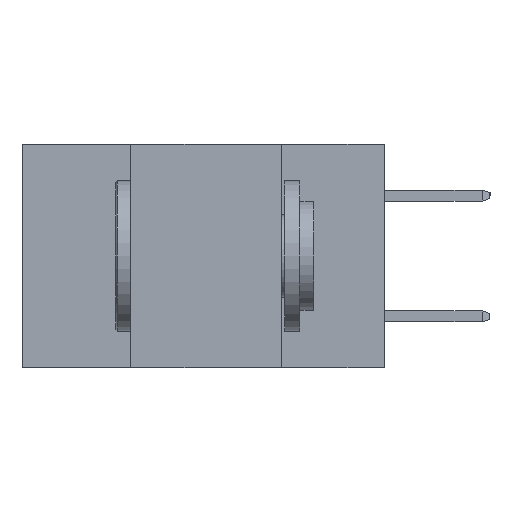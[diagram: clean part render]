
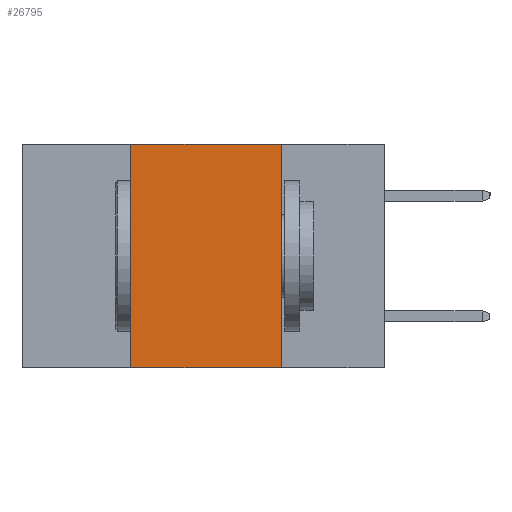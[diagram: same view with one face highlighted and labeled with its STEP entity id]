
A CAD part, left-side view. The second image highlights one B-rep face of the part: STEP entity #26795.
In plain terms, the highlighted planar face has unit normal (-1, 0, 0).
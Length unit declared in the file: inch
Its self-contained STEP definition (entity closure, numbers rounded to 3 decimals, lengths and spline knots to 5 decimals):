
#419 = CARTESIAN_POINT ( 'NONE',  ( 0., 0.17, -0.37 ) ) ;
#626 = VECTOR ( 'NONE', #10314, 39.37008 ) ;
#770 = DIRECTION ( 'NONE',  ( 0., 0., -1. ) ) ;
#1267 = EDGE_LOOP ( 'NONE', ( #12982, #4281, #22474, #10331 ) ) ;
#1413 = VECTOR ( 'NONE', #6428, 39.37008 ) ;
#2016 = VECTOR ( 'NONE', #3237, 39.37008 ) ;
#3237 = DIRECTION ( 'NONE',  ( 0., 0., -1. ) ) ;
#4281 = ORIENTED_EDGE ( 'NONE', *, *, #20757, .F. ) ;
#4662 = EDGE_CURVE ( 'NONE', #10327, #23945, #9200, .T. ) ;
#4776 = VECTOR ( 'NONE', #5690, 39.37008 ) ;
#4963 = FACE_OUTER_BOUND ( 'NONE', #1267, .T. ) ;
#5690 = DIRECTION ( 'NONE',  ( 0., 0., 1. ) ) ;
#6217 = LINE ( 'NONE', #24453, #4776 ) ;
#6428 = DIRECTION ( 'NONE',  ( 0., -1., 0. ) ) ;
#6830 = CARTESIAN_POINT ( 'NONE',  ( 0., 0.6, -0.37 ) ) ;
#9200 = LINE ( 'NONE', #15189, #2016 ) ;
#10174 = CARTESIAN_POINT ( 'NONE',  ( 0., 0.6, 0. ) ) ;
#10314 = DIRECTION ( 'NONE',  ( 0., -1., 0. ) ) ;
#10327 = VERTEX_POINT ( 'NONE', #24764 ) ;
#10331 = ORIENTED_EDGE ( 'NONE', *, *, #12918, .T. ) ;
#10918 = CARTESIAN_POINT ( 'NONE',  ( 0., 0.42, -0.37 ) ) ;
#12217 = CARTESIAN_POINT ( 'NONE',  ( 0., 0.42, 0. ) ) ;
#12918 = EDGE_CURVE ( 'NONE', #22150, #23945, #21374, .T. ) ;
#12982 = ORIENTED_EDGE ( 'NONE', *, *, #4662, .F. ) ;
#15034 = DIRECTION ( 'NONE',  ( 1., 0., 0. ) ) ;
#15127 = VERTEX_POINT ( 'NONE', #12217 ) ;
#15145 = EDGE_CURVE ( 'NONE', #22150, #15127, #6217, .T. ) ;
#15189 = CARTESIAN_POINT ( 'NONE',  ( 0., 0.17, -0.37 ) ) ;
#20757 = EDGE_CURVE ( 'NONE', #15127, #10327, #25006, .T. ) ;
#21374 = LINE ( 'NONE', #6830, #1413 ) ;
#21423 = PLANE ( 'NONE',  #23201 ) ;
#22150 = VERTEX_POINT ( 'NONE', #10918 ) ;
#22474 = ORIENTED_EDGE ( 'NONE', *, *, #15145, .F. ) ;
#23201 = AXIS2_PLACEMENT_3D ( 'NONE', #23736, #15034, #770 ) ;
#23736 = CARTESIAN_POINT ( 'NONE',  ( 0., 0.6, 0. ) ) ;
#23945 = VERTEX_POINT ( 'NONE', #419 ) ;
#24453 = CARTESIAN_POINT ( 'NONE',  ( 0., 0.42, -0.37 ) ) ;
#24764 = CARTESIAN_POINT ( 'NONE',  ( 0., 0.17, 0. ) ) ;
#25006 = LINE ( 'NONE', #10174, #626 ) ;
#26795 = ADVANCED_FACE ( 'NONE', ( #4963 ), #21423, .F. ) ;
